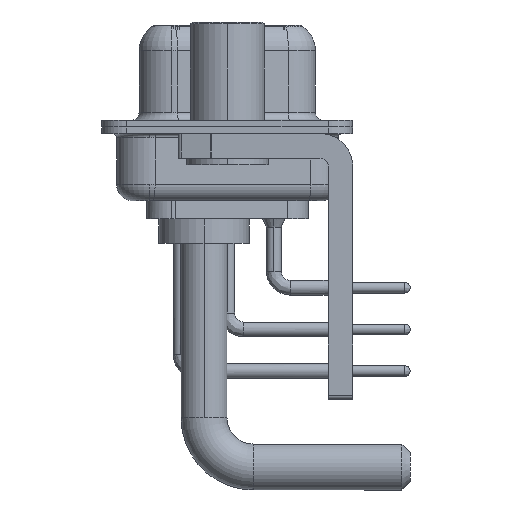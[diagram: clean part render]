
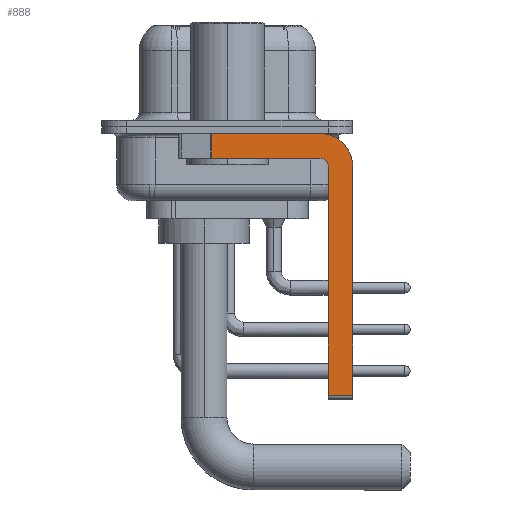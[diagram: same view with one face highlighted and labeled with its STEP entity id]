
A CAD part, left-side view. The second image highlights one B-rep face of the part: STEP entity #888.
In plain terms, the highlighted planar face has unit normal (-1, 0, 0).
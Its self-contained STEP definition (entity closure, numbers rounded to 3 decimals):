
#624 = CIRCLE ( 'NONE', #4590, 2. ) ;
#888 = ADVANCED_FACE ( 'NONE', ( #20610 ), #6557, .F. ) ;
#2142 = DIRECTION ( 'NONE',  ( 0., 0., 1. ) ) ;
#2683 = VERTEX_POINT ( 'NONE', #8831 ) ;
#3806 = VECTOR ( 'NONE', #17537, 1000. ) ;
#3878 = VERTEX_POINT ( 'NONE', #4962 ) ;
#4406 = VECTOR ( 'NONE', #29523, 1000. ) ;
#4590 = AXIS2_PLACEMENT_3D ( 'NONE', #10208, #18911, #5398 ) ;
#4936 = ORIENTED_EDGE ( 'NONE', *, *, #24292, .F. ) ;
#4962 = CARTESIAN_POINT ( 'NONE',  ( -2.9, -6.15, -16.35 ) ) ;
#5005 = DIRECTION ( 'NONE',  ( 0., 0., 1. ) ) ;
#5398 = DIRECTION ( 'NONE',  ( 0., 0., -1. ) ) ;
#5628 = CARTESIAN_POINT ( 'NONE',  ( -2.9, -6.15, -2.4 ) ) ;
#5897 = CARTESIAN_POINT ( 'NONE',  ( -2.9, 3., -0.4 ) ) ;
#6557 = PLANE ( 'NONE',  #28216 ) ;
#6702 = LINE ( 'NONE', #17719, #3806 ) ;
#7663 = CARTESIAN_POINT ( 'NONE',  ( -2.9, -6.15, -16.6 ) ) ;
#8034 = CARTESIAN_POINT ( 'NONE',  ( -2.9, 0.978, -0.4 ) ) ;
#8377 = EDGE_LOOP ( 'NONE', ( #34814, #17298, #4936, #31750, #27931, #20275, #23158, #26297 ) ) ;
#8449 = EDGE_CURVE ( 'NONE', #3878, #8932, #6702, .T. ) ;
#8831 = CARTESIAN_POINT ( 'NONE',  ( -2.9, -5.65, -1.9 ) ) ;
#8932 = VERTEX_POINT ( 'NONE', #9502 ) ;
#9237 = DIRECTION ( 'NONE',  ( 0., 0., -1. ) ) ;
#9502 = CARTESIAN_POINT ( 'NONE',  ( -2.9, -7.65, -16.35 ) ) ;
#10208 = CARTESIAN_POINT ( 'NONE',  ( -2.9, -5.65, -2.4 ) ) ;
#10305 = CARTESIAN_POINT ( 'NONE',  ( -2.9, -5.65, -2.4 ) ) ;
#10752 = CARTESIAN_POINT ( 'NONE',  ( -2.9, -5.65, -1.9 ) ) ;
#10881 = LINE ( 'NONE', #24563, #4406 ) ;
#11160 = VERTEX_POINT ( 'NONE', #26011 ) ;
#12704 = EDGE_CURVE ( 'NONE', #30924, #11160, #30369, .T. ) ;
#14121 = LINE ( 'NONE', #10752, #28428 ) ;
#14359 = EDGE_CURVE ( 'NONE', #11160, #18658, #624, .T. ) ;
#14755 = VECTOR ( 'NONE', #27211, 1000. ) ;
#14919 = CARTESIAN_POINT ( 'NONE',  ( -2.9, -5.65, -2.4 ) ) ;
#15540 = EDGE_CURVE ( 'NONE', #29854, #2683, #22823, .T. ) ;
#17298 = ORIENTED_EDGE ( 'NONE', *, *, #33637, .T. ) ;
#17537 = DIRECTION ( 'NONE',  ( 0., -1., 0. ) ) ;
#17719 = CARTESIAN_POINT ( 'NONE',  ( -2.9, -5.65, -16.35 ) ) ;
#18658 = VERTEX_POINT ( 'NONE', #31051 ) ;
#18911 = DIRECTION ( 'NONE',  ( 1., 0., 0. ) ) ;
#18915 = CARTESIAN_POINT ( 'NONE',  ( -2.9, 0.978, -1.9 ) ) ;
#19289 = DIRECTION ( 'NONE',  ( 0., 1., 0. ) ) ;
#20275 = ORIENTED_EDGE ( 'NONE', *, *, #8449, .T. ) ;
#20610 = FACE_OUTER_BOUND ( 'NONE', #8377, .T. ) ;
#20636 = EDGE_CURVE ( 'NONE', #18658, #8932, #10881, .T. ) ;
#20973 = EDGE_CURVE ( 'NONE', #3878, #29854, #26492, .T. ) ;
#22823 = CIRCLE ( 'NONE', #34141, 0.5 ) ;
#22915 = DIRECTION ( 'NONE',  ( 1., 0., 0. ) ) ;
#22934 = LINE ( 'NONE', #27891, #24663 ) ;
#23158 = ORIENTED_EDGE ( 'NONE', *, *, #20636, .F. ) ;
#24292 = EDGE_CURVE ( 'NONE', #2683, #33074, #14121, .T. ) ;
#24563 = CARTESIAN_POINT ( 'NONE',  ( -2.9, -7.65, -2.4 ) ) ;
#24663 = VECTOR ( 'NONE', #28406, 1000. ) ;
#26011 = CARTESIAN_POINT ( 'NONE',  ( -2.9, -5.65, -0.4 ) ) ;
#26297 = ORIENTED_EDGE ( 'NONE', *, *, #14359, .F. ) ;
#26492 = LINE ( 'NONE', #7663, #29921 ) ;
#27211 = DIRECTION ( 'NONE',  ( 0., -1., 0. ) ) ;
#27891 = CARTESIAN_POINT ( 'NONE',  ( -2.9, 0.978, -1.9 ) ) ;
#27931 = ORIENTED_EDGE ( 'NONE', *, *, #20973, .F. ) ;
#28216 = AXIS2_PLACEMENT_3D ( 'NONE', #14919, #22915, #9237 ) ;
#28406 = DIRECTION ( 'NONE',  ( 0., 0., -1. ) ) ;
#28428 = VECTOR ( 'NONE', #19289, 1000. ) ;
#29523 = DIRECTION ( 'NONE',  ( 0., 0., -1. ) ) ;
#29854 = VERTEX_POINT ( 'NONE', #5628 ) ;
#29921 = VECTOR ( 'NONE', #5005, 1000. ) ;
#30369 = LINE ( 'NONE', #5897, #14755 ) ;
#30924 = VERTEX_POINT ( 'NONE', #8034 ) ;
#31051 = CARTESIAN_POINT ( 'NONE',  ( -2.9, -7.65, -2.4 ) ) ;
#31750 = ORIENTED_EDGE ( 'NONE', *, *, #15540, .F. ) ;
#33074 = VERTEX_POINT ( 'NONE', #18915 ) ;
#33637 = EDGE_CURVE ( 'NONE', #30924, #33074, #22934, .T. ) ;
#34141 = AXIS2_PLACEMENT_3D ( 'NONE', #10305, #34763, #2142 ) ;
#34763 = DIRECTION ( 'NONE',  ( -1., 0., 0. ) ) ;
#34814 = ORIENTED_EDGE ( 'NONE', *, *, #12704, .F. ) ;
